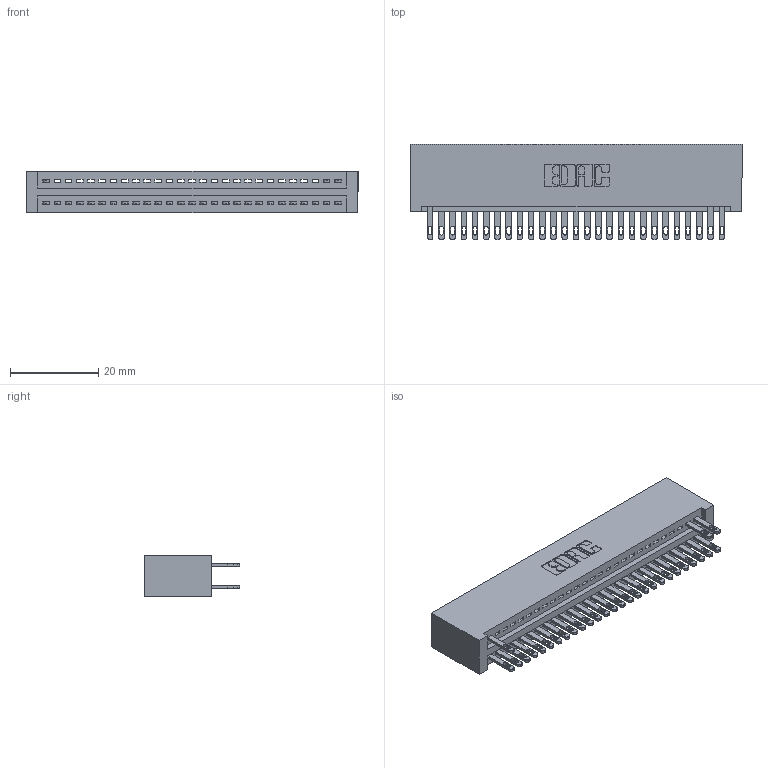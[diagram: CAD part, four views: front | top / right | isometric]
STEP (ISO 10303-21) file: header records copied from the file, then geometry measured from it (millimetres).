
FILE_DESCRIPTION (( 'STEP AP203' ), '1' );
FILE_NAME ('345-054-500-201.STEP', '2018-09-23T19:35:47', ( '' ), ( '' ), 'SwSTEP 2.0', 'SolidWorks 2016', '' );
FILE_SCHEMA (( 'CONFIG_CONTROL_DESIGN' ));
Length unit declared in the file: inch
Products named in the file (3): 345 Part_No Mounting Lugs; 345-292-001_345-293-100; 345-054-500-201
Assembly tree (31 placements, depth 2):
  345-054-500-201
    345 Part_No Mounting Lugs
    345-292-001_345-293-100  x30
Bounding box: 75.18 x 21.51 x 9.4 mm (x, y, z)
Volume: 7655.5 mm3; surface area: 10409.5 mm2
Topology: 31 solids, 31 shells, 1690 faces, 5195 edges, 3462 vertices
Faces by surface type: plane 1054, cylinder 636
Entity records: 22089 total; most frequent: CARTESIAN_POINT 3820, ORIENTED_EDGE 3778, DIRECTION 3357, EDGE_CURVE 1889, LINE 1653, VECTOR 1653, VERTEX_POINT 1258, AXIS2_PLACEMENT_3D 852
